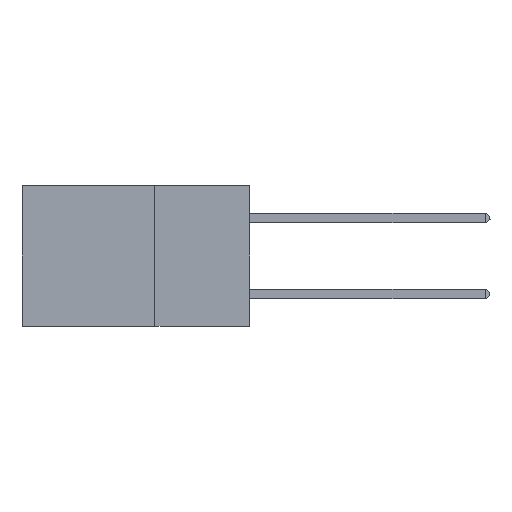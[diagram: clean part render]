
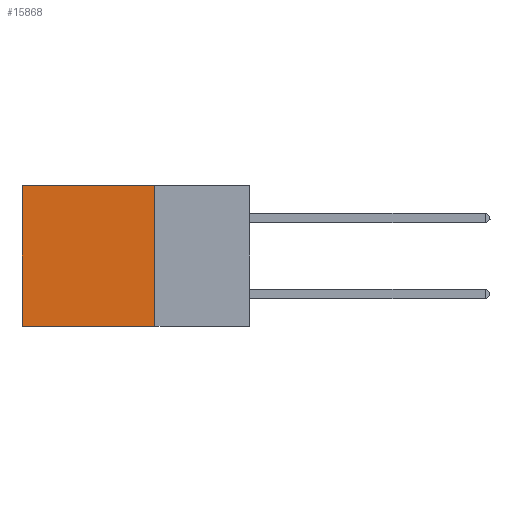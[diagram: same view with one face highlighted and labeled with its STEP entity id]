
A CAD part, left-side view. The second image highlights one B-rep face of the part: STEP entity #15868.
In plain terms, the highlighted planar face has unit normal (-1, 0, 0).
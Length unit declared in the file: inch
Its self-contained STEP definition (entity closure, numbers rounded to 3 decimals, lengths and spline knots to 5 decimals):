
#964 = CARTESIAN_POINT ( 'NONE',  ( 0.2875, 0.6, -0.37 ) ) ;
#1922 = CARTESIAN_POINT ( 'NONE',  ( 0.2875, 0.6, 0. ) ) ;
#2235 = LINE ( 'NONE', #21433, #5364 ) ;
#3926 = DIRECTION ( 'NONE',  ( 0., 1., 0. ) ) ;
#4314 = EDGE_CURVE ( 'NONE', #8505, #15292, #2235, .T. ) ;
#5111 = DIRECTION ( 'NONE',  ( 0., 1., 0. ) ) ;
#5364 = VECTOR ( 'NONE', #5111, 39.37008 ) ;
#5790 = LINE ( 'NONE', #6859, #7661 ) ;
#6859 = CARTESIAN_POINT ( 'NONE',  ( 0.2875, 0.25, 0. ) ) ;
#7661 = VECTOR ( 'NONE', #20772, 39.37008 ) ;
#8505 = VERTEX_POINT ( 'NONE', #24553 ) ;
#10729 = ORIENTED_EDGE ( 'NONE', *, *, #21805, .T. ) ;
#10870 = ORIENTED_EDGE ( 'NONE', *, *, #22173, .T. ) ;
#13139 = CARTESIAN_POINT ( 'NONE',  ( 0.2875, 0.25, 0. ) ) ;
#14648 = ORIENTED_EDGE ( 'NONE', *, *, #19110, .F. ) ;
#15041 = DIRECTION ( 'NONE',  ( 1., 0., 0. ) ) ;
#15292 = VERTEX_POINT ( 'NONE', #964 ) ;
#15363 = AXIS2_PLACEMENT_3D ( 'NONE', #13139, #15041, #17119 ) ;
#15577 = FACE_OUTER_BOUND ( 'NONE', #22056, .T. ) ;
#15868 = ADVANCED_FACE ( 'NONE', ( #15577 ), #17046, .F. ) ;
#17046 = PLANE ( 'NONE',  #15363 ) ;
#17076 = LINE ( 'NONE', #18611, #22041 ) ;
#17119 = DIRECTION ( 'NONE',  ( 0., 0., -1. ) ) ;
#18611 = CARTESIAN_POINT ( 'NONE',  ( 0.2875, 0.6, 0. ) ) ;
#19110 = EDGE_CURVE ( 'NONE', #21846, #8505, #5790, .T. ) ;
#19591 = LINE ( 'NONE', #22076, #22365 ) ;
#20481 = VERTEX_POINT ( 'NONE', #1922 ) ;
#20772 = DIRECTION ( 'NONE',  ( 0., 0., -1. ) ) ;
#21433 = CARTESIAN_POINT ( 'NONE',  ( 0.2875, 0.25, -0.37 ) ) ;
#21805 = EDGE_CURVE ( 'NONE', #21846, #20481, #19591, .T. ) ;
#21833 = ORIENTED_EDGE ( 'NONE', *, *, #4314, .F. ) ;
#21846 = VERTEX_POINT ( 'NONE', #21909 ) ;
#21909 = CARTESIAN_POINT ( 'NONE',  ( 0.2875, 0.25, 0. ) ) ;
#22041 = VECTOR ( 'NONE', #24585, 39.37008 ) ;
#22056 = EDGE_LOOP ( 'NONE', ( #10870, #21833, #14648, #10729 ) ) ;
#22076 = CARTESIAN_POINT ( 'NONE',  ( 0.2875, 0.25, 0. ) ) ;
#22173 = EDGE_CURVE ( 'NONE', #20481, #15292, #17076, .T. ) ;
#22365 = VECTOR ( 'NONE', #3926, 39.37008 ) ;
#24553 = CARTESIAN_POINT ( 'NONE',  ( 0.2875, 0.25, -0.37 ) ) ;
#24585 = DIRECTION ( 'NONE',  ( 0., 0., -1. ) ) ;
